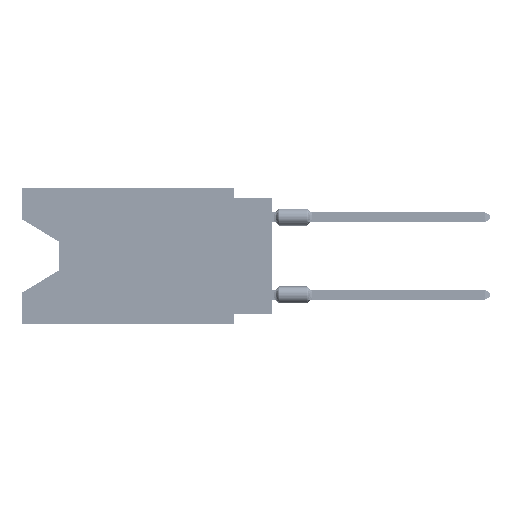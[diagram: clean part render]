
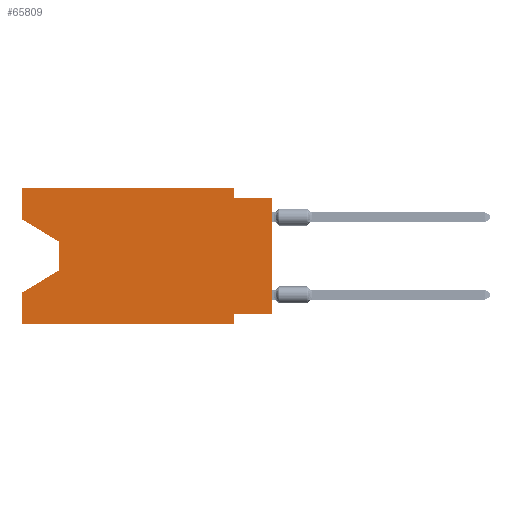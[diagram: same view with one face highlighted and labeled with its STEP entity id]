
A CAD part, left-side view. The second image highlights one B-rep face of the part: STEP entity #65809.
In plain terms, the highlighted planar face has unit normal (-1, 0, 0).
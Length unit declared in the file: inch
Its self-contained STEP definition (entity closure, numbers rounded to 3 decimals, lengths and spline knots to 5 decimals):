
#2762 = CARTESIAN_POINT ( 'NONE',  ( 0., 0., 0. ) ) ;
#2862 = PLANE ( 'NONE',  #65340 ) ;
#3122 = VECTOR ( 'NONE', #92290, 39.37008 ) ;
#3227 = CARTESIAN_POINT ( 'NONE',  ( 0., 0.645, 0. ) ) ;
#4316 = CARTESIAN_POINT ( 'NONE',  ( 0., 0.645, 0. ) ) ;
#5074 = LINE ( 'NONE', #94901, #42297 ) ;
#5751 = DIRECTION ( 'NONE',  ( 0., 0., 1. ) ) ;
#8157 = ORIENTED_EDGE ( 'NONE', *, *, #41571, .T. ) ;
#9379 = CARTESIAN_POINT ( 'NONE',  ( 0., 0.55, -0.212 ) ) ;
#10709 = DIRECTION ( 'NONE',  ( 0., 0., -1. ) ) ;
#11199 = CARTESIAN_POINT ( 'NONE',  ( 0., 0.645, 0. ) ) ;
#11744 = ORIENTED_EDGE ( 'NONE', *, *, #33135, .T. ) ;
#12117 = DIRECTION ( 'NONE',  ( 0., 0., -1. ) ) ;
#12705 = ORIENTED_EDGE ( 'NONE', *, *, #16875, .F. ) ;
#12772 = VECTOR ( 'NONE', #39094, 39.37008 ) ;
#12832 = VECTOR ( 'NONE', #84872, 39.37008 ) ;
#14570 = CARTESIAN_POINT ( 'NONE',  ( 0., 0.1, -0.35 ) ) ;
#14855 = DIRECTION ( 'NONE',  ( 0., -1., 0. ) ) ;
#14979 = ORIENTED_EDGE ( 'NONE', *, *, #74989, .F. ) ;
#15648 = CARTESIAN_POINT ( 'NONE',  ( 0., 0.55, -0.138 ) ) ;
#16875 = EDGE_CURVE ( 'NONE', #35097, #51879, #66104, .T. ) ;
#18563 = DIRECTION ( 'NONE',  ( 1., 0., 0. ) ) ;
#21888 = CARTESIAN_POINT ( 'NONE',  ( 0., 0., -0.325 ) ) ;
#22522 = VERTEX_POINT ( 'NONE', #33533 ) ;
#23882 = DIRECTION ( 'NONE',  ( 0., 0., 1. ) ) ;
#23943 = VERTEX_POINT ( 'NONE', #51637 ) ;
#24406 = VECTOR ( 'NONE', #70525, 39.37008 ) ;
#24914 = CARTESIAN_POINT ( 'NONE',  ( 0., 0., -0.025 ) ) ;
#25635 = EDGE_LOOP ( 'NONE', ( #27414, #8157, #48449, #64400, #11744, #29388, #47027, #72294, #14979, #85902, #45570, #12705 ) ) ;
#26568 = EDGE_CURVE ( 'NONE', #84786, #36627, #38099, .T. ) ;
#27314 = LINE ( 'NONE', #72438, #59886 ) ;
#27414 = ORIENTED_EDGE ( 'NONE', *, *, #70388, .T. ) ;
#29388 = ORIENTED_EDGE ( 'NONE', *, *, #90289, .F. ) ;
#33135 = EDGE_CURVE ( 'NONE', #47995, #51691, #84371, .T. ) ;
#33533 = CARTESIAN_POINT ( 'NONE',  ( 0., 0.1, -0.025 ) ) ;
#35097 = VERTEX_POINT ( 'NONE', #54300 ) ;
#35791 = LINE ( 'NONE', #45247, #45154 ) ;
#36627 = VERTEX_POINT ( 'NONE', #37526 ) ;
#37526 = CARTESIAN_POINT ( 'NONE',  ( 0., 0., -0.025 ) ) ;
#37698 = CARTESIAN_POINT ( 'NONE',  ( 0., 0.1, 0. ) ) ;
#38099 = LINE ( 'NONE', #2762, #52283 ) ;
#39094 = DIRECTION ( 'NONE',  ( 0., 0.855, -0.519 ) ) ;
#41156 = CARTESIAN_POINT ( 'NONE',  ( 0., 0.1, -0.35 ) ) ;
#41571 = EDGE_CURVE ( 'NONE', #70644, #72805, #90596, .T. ) ;
#42297 = VECTOR ( 'NONE', #66378, 39.37008 ) ;
#45154 = VECTOR ( 'NONE', #66202, 39.37008 ) ;
#45247 = CARTESIAN_POINT ( 'NONE',  ( 0., 0.645, 0. ) ) ;
#45570 = ORIENTED_EDGE ( 'NONE', *, *, #50916, .F. ) ;
#47027 = ORIENTED_EDGE ( 'NONE', *, *, #82159, .F. ) ;
#47995 = VERTEX_POINT ( 'NONE', #90765 ) ;
#48449 = ORIENTED_EDGE ( 'NONE', *, *, #89477, .T. ) ;
#49743 = LINE ( 'NONE', #56132, #12772 ) ;
#50916 = EDGE_CURVE ( 'NONE', #51879, #80554, #82994, .T. ) ;
#51637 = CARTESIAN_POINT ( 'NONE',  ( 0., 0.645, -0.26975 ) ) ;
#51691 = VERTEX_POINT ( 'NONE', #14570 ) ;
#51879 = VERTEX_POINT ( 'NONE', #3227 ) ;
#52283 = VECTOR ( 'NONE', #23882, 39.37008 ) ;
#52920 = CARTESIAN_POINT ( 'NONE',  ( 0., 0.1, -0.325 ) ) ;
#53277 = CARTESIAN_POINT ( 'NONE',  ( 0., 0.55, -0.138 ) ) ;
#54146 = VECTOR ( 'NONE', #14855, 39.37008 ) ;
#54300 = CARTESIAN_POINT ( 'NONE',  ( 0., 0.645, -0.08025 ) ) ;
#55410 = LINE ( 'NONE', #41156, #12832 ) ;
#56132 = CARTESIAN_POINT ( 'NONE',  ( 0., 0.55, -0.212 ) ) ;
#58089 = EDGE_CURVE ( 'NONE', #47995, #23943, #35791, .T. ) ;
#59886 = VECTOR ( 'NONE', #12117, 39.37008 ) ;
#60899 = CARTESIAN_POINT ( 'NONE',  ( 0., 0.645, 0. ) ) ;
#61785 = VERTEX_POINT ( 'NONE', #52920 ) ;
#64400 = ORIENTED_EDGE ( 'NONE', *, *, #58089, .F. ) ;
#65340 = AXIS2_PLACEMENT_3D ( 'NONE', #11199, #18563, #10709 ) ;
#65809 = ADVANCED_FACE ( 'NONE', ( #70564 ), #2862, .F. ) ;
#66104 = LINE ( 'NONE', #4316, #76387 ) ;
#66202 = DIRECTION ( 'NONE',  ( 0., 0., 1. ) ) ;
#66378 = DIRECTION ( 'NONE',  ( 0., 1., 0. ) ) ;
#69689 = CARTESIAN_POINT ( 'NONE',  ( 0., 0.645, -0.08025 ) ) ;
#70388 = EDGE_CURVE ( 'NONE', #35097, #70644, #92767, .T. ) ;
#70525 = DIRECTION ( 'NONE',  ( 0., -1., 0. ) ) ;
#70564 = FACE_OUTER_BOUND ( 'NONE', #25635, .T. ) ;
#70644 = VERTEX_POINT ( 'NONE', #15648 ) ;
#72294 = ORIENTED_EDGE ( 'NONE', *, *, #26568, .T. ) ;
#72438 = CARTESIAN_POINT ( 'NONE',  ( 0., 0.1, 0. ) ) ;
#72805 = VERTEX_POINT ( 'NONE', #9379 ) ;
#74989 = EDGE_CURVE ( 'NONE', #22522, #36627, #92150, .T. ) ;
#76387 = VECTOR ( 'NONE', #5751, 39.37008 ) ;
#80554 = VERTEX_POINT ( 'NONE', #37698 ) ;
#81594 = CARTESIAN_POINT ( 'NONE',  ( 0., 0.645, -0.35 ) ) ;
#82159 = EDGE_CURVE ( 'NONE', #84786, #61785, #5074, .T. ) ;
#82994 = LINE ( 'NONE', #60899, #89895 ) ;
#83476 = DIRECTION ( 'NONE',  ( 0., -1., 0. ) ) ;
#84371 = LINE ( 'NONE', #81594, #54146 ) ;
#84786 = VERTEX_POINT ( 'NONE', #21888 ) ;
#84872 = DIRECTION ( 'NONE',  ( 0., 0., -1. ) ) ;
#85902 = ORIENTED_EDGE ( 'NONE', *, *, #90855, .F. ) ;
#86387 = VECTOR ( 'NONE', #90105, 39.37008 ) ;
#89477 = EDGE_CURVE ( 'NONE', #72805, #23943, #49743, .T. ) ;
#89895 = VECTOR ( 'NONE', #83476, 39.37008 ) ;
#90105 = DIRECTION ( 'NONE',  ( 0., 0., -1. ) ) ;
#90289 = EDGE_CURVE ( 'NONE', #61785, #51691, #55410, .T. ) ;
#90596 = LINE ( 'NONE', #53277, #86387 ) ;
#90765 = CARTESIAN_POINT ( 'NONE',  ( 0., 0.645, -0.35 ) ) ;
#90855 = EDGE_CURVE ( 'NONE', #80554, #22522, #27314, .T. ) ;
#92150 = LINE ( 'NONE', #24914, #24406 ) ;
#92290 = DIRECTION ( 'NONE',  ( 0., -0.855, -0.519 ) ) ;
#92767 = LINE ( 'NONE', #69689, #3122 ) ;
#94901 = CARTESIAN_POINT ( 'NONE',  ( 0., 0., -0.325 ) ) ;
